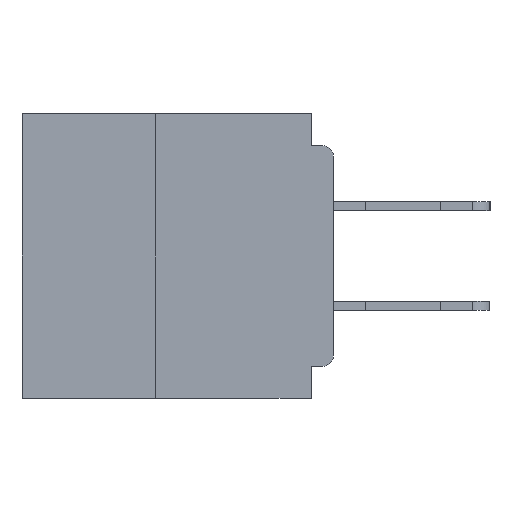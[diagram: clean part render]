
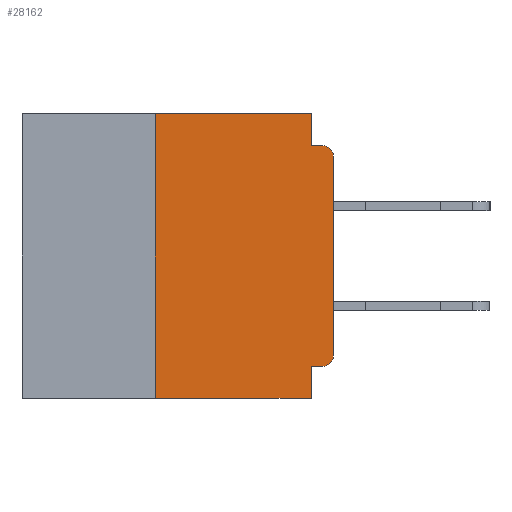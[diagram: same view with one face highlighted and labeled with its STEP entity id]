
A CAD part, left-side view. The second image highlights one B-rep face of the part: STEP entity #28162.
In plain terms, the highlighted planar face has unit normal (-1, 0, 0).
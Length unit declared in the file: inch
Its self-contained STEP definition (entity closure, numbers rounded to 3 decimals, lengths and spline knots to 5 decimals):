
#1614 = DIRECTION ( 'NONE',  ( -1., 0., 0. ) ) ;
#2502 = CARTESIAN_POINT ( 'NONE',  ( 0., 0.25, -0.4 ) ) ;
#2806 = DIRECTION ( 'NONE',  ( 0., 1., 0. ) ) ;
#4616 = VECTOR ( 'NONE', #26259, 39.37008 ) ;
#5115 = EDGE_CURVE ( 'NONE', #40894, #31740, #28693, .T. ) ;
#5855 = LINE ( 'NONE', #45874, #4616 ) ;
#6149 = CARTESIAN_POINT ( 'NONE',  ( 0., 0.25, 0. ) ) ;
#6733 = DIRECTION ( 'NONE',  ( 0., 0., 1. ) ) ;
#8236 = AXIS2_PLACEMENT_3D ( 'NONE', #42791, #19208, #46724 ) ;
#8297 = CARTESIAN_POINT ( 'NONE',  ( 0., 0.031, -0.045 ) ) ;
#8581 = CIRCLE ( 'NONE', #42203, 0.015 ) ;
#9159 = CIRCLE ( 'NONE', #8236, 0.015 ) ;
#10637 = VECTOR ( 'NONE', #39724, 39.37008 ) ;
#10721 = DIRECTION ( 'NONE',  ( 0., -1., 0. ) ) ;
#10787 = EDGE_CURVE ( 'NONE', #31512, #18968, #48478, .T. ) ;
#11160 = PLANE ( 'NONE',  #35872 ) ;
#11454 = ORIENTED_EDGE ( 'NONE', *, *, #22879, .F. ) ;
#11791 = ORIENTED_EDGE ( 'NONE', *, *, #10787, .T. ) ;
#12011 = EDGE_CURVE ( 'NONE', #31512, #16401, #5855, .T. ) ;
#14277 = VERTEX_POINT ( 'NONE', #44656 ) ;
#15200 = EDGE_CURVE ( 'NONE', #19177, #27242, #19769, .T. ) ;
#15426 = VERTEX_POINT ( 'NONE', #42769 ) ;
#16076 = CARTESIAN_POINT ( 'NONE',  ( 0., 0.031, 0. ) ) ;
#16401 = VERTEX_POINT ( 'NONE', #6149 ) ;
#17341 = CARTESIAN_POINT ( 'NONE',  ( 0., 0.015, -0.045 ) ) ;
#18483 = CARTESIAN_POINT ( 'NONE',  ( 0., 0., 0. ) ) ;
#18968 = VERTEX_POINT ( 'NONE', #38663 ) ;
#19177 = VERTEX_POINT ( 'NONE', #8297 ) ;
#19208 = DIRECTION ( 'NONE',  ( -1., 0., 0. ) ) ;
#19769 = LINE ( 'NONE', #25593, #49884 ) ;
#20218 = ORIENTED_EDGE ( 'NONE', *, *, #38723, .F. ) ;
#22334 = ORIENTED_EDGE ( 'NONE', *, *, #49873, .F. ) ;
#22879 = EDGE_CURVE ( 'NONE', #31740, #18968, #40736, .T. ) ;
#23115 = DIRECTION ( 'NONE',  ( 0., 0., -1. ) ) ;
#25225 = CARTESIAN_POINT ( 'NONE',  ( 0., 0.015, -0.34 ) ) ;
#25275 = ORIENTED_EDGE ( 'NONE', *, *, #15200, .F. ) ;
#25593 = CARTESIAN_POINT ( 'NONE',  ( 0., 0., -0.045 ) ) ;
#26259 = DIRECTION ( 'NONE',  ( 0., 0., 1. ) ) ;
#26398 = EDGE_LOOP ( 'NONE', ( #38085, #41509, #25275, #20218, #22334, #28500, #11791, #11454, #35933, #44903 ) ) ;
#27242 = VERTEX_POINT ( 'NONE', #17341 ) ;
#28162 = ADVANCED_FACE ( 'NONE', ( #41569 ), #11160, .F. ) ;
#28500 = ORIENTED_EDGE ( 'NONE', *, *, #12011, .F. ) ;
#28693 = LINE ( 'NONE', #34339, #36694 ) ;
#28815 = VECTOR ( 'NONE', #10721, 39.37008 ) ;
#29195 = DIRECTION ( 'NONE',  ( 0., 0., -1. ) ) ;
#29686 = CARTESIAN_POINT ( 'NONE',  ( 0., 0.031, -0.4 ) ) ;
#31512 = VERTEX_POINT ( 'NONE', #2502 ) ;
#31674 = EDGE_CURVE ( 'NONE', #15426, #27242, #9159, .T. ) ;
#31740 = VERTEX_POINT ( 'NONE', #43132 ) ;
#33501 = DIRECTION ( 'NONE',  ( 0., -1., 0. ) ) ;
#33927 = VECTOR ( 'NONE', #46570, 39.37008 ) ;
#34023 = VECTOR ( 'NONE', #6733, 39.37008 ) ;
#34339 = CARTESIAN_POINT ( 'NONE',  ( 0., 0., -0.355 ) ) ;
#34720 = CARTESIAN_POINT ( 'NONE',  ( 0., 0.437, 0. ) ) ;
#35245 = LINE ( 'NONE', #18483, #34023 ) ;
#35872 = AXIS2_PLACEMENT_3D ( 'NONE', #38621, #46664, #23115 ) ;
#35933 = ORIENTED_EDGE ( 'NONE', *, *, #5115, .F. ) ;
#36694 = VECTOR ( 'NONE', #2806, 39.37008 ) ;
#38085 = ORIENTED_EDGE ( 'NONE', *, *, #49005, .T. ) ;
#38621 = CARTESIAN_POINT ( 'NONE',  ( 0., 0.437, 0. ) ) ;
#38663 = CARTESIAN_POINT ( 'NONE',  ( 0., 0.031, -0.4 ) ) ;
#38723 = EDGE_CURVE ( 'NONE', #42416, #19177, #39677, .T. ) ;
#39677 = LINE ( 'NONE', #16076, #10637 ) ;
#39724 = DIRECTION ( 'NONE',  ( 0., 0., -1. ) ) ;
#40736 = LINE ( 'NONE', #29686, #49872 ) ;
#40894 = VERTEX_POINT ( 'NONE', #41757 ) ;
#41509 = ORIENTED_EDGE ( 'NONE', *, *, #31674, .T. ) ;
#41568 = DIRECTION ( 'NONE',  ( 0., 0., -1. ) ) ;
#41569 = FACE_OUTER_BOUND ( 'NONE', #26398, .T. ) ;
#41757 = CARTESIAN_POINT ( 'NONE',  ( 0., 0.015, -0.355 ) ) ;
#42203 = AXIS2_PLACEMENT_3D ( 'NONE', #25225, #1614, #29195 ) ;
#42291 = CARTESIAN_POINT ( 'NONE',  ( 0., 0.437, -0.4 ) ) ;
#42416 = VERTEX_POINT ( 'NONE', #44585 ) ;
#42769 = CARTESIAN_POINT ( 'NONE',  ( 0., 0., -0.06 ) ) ;
#42791 = CARTESIAN_POINT ( 'NONE',  ( 0., 0.015, -0.06 ) ) ;
#43132 = CARTESIAN_POINT ( 'NONE',  ( 0., 0.031, -0.355 ) ) ;
#44585 = CARTESIAN_POINT ( 'NONE',  ( 0., 0.031, 0. ) ) ;
#44656 = CARTESIAN_POINT ( 'NONE',  ( 0., 0., -0.34 ) ) ;
#44903 = ORIENTED_EDGE ( 'NONE', *, *, #50201, .T. ) ;
#45625 = LINE ( 'NONE', #34720, #33927 ) ;
#45874 = CARTESIAN_POINT ( 'NONE',  ( 0., 0.25, -0.4 ) ) ;
#46570 = DIRECTION ( 'NONE',  ( 0., -1., 0. ) ) ;
#46664 = DIRECTION ( 'NONE',  ( 1., 0., 0. ) ) ;
#46724 = DIRECTION ( 'NONE',  ( 0., 0., -1. ) ) ;
#48478 = LINE ( 'NONE', #42291, #28815 ) ;
#49005 = EDGE_CURVE ( 'NONE', #14277, #15426, #35245, .T. ) ;
#49872 = VECTOR ( 'NONE', #41568, 39.37008 ) ;
#49873 = EDGE_CURVE ( 'NONE', #16401, #42416, #45625, .T. ) ;
#49884 = VECTOR ( 'NONE', #33501, 39.37008 ) ;
#50201 = EDGE_CURVE ( 'NONE', #40894, #14277, #8581, .T. ) ;
